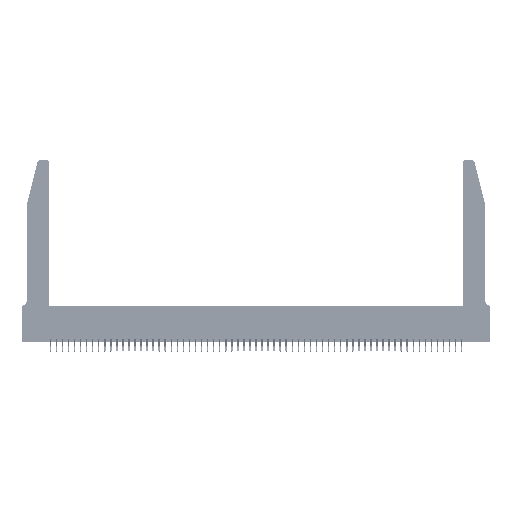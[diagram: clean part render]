
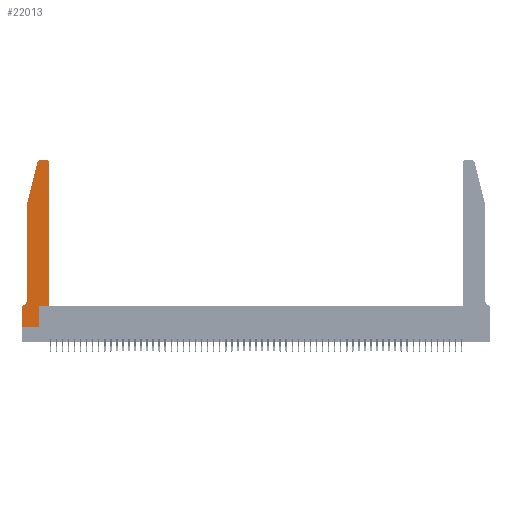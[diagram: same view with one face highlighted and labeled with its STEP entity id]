
A CAD part, top view. The second image highlights one B-rep face of the part: STEP entity #22013.
In plain terms, the highlighted planar face has unit normal (0, 0, 1).
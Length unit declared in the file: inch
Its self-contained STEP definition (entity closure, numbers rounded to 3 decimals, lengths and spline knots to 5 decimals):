
#356 = VERTEX_POINT ( 'NONE', #2509 ) ;
#990 = DIRECTION ( 'NONE',  ( 1., 0., 0. ) ) ;
#1100 = VECTOR ( 'NONE', #45764, 39.37008 ) ;
#1460 = FACE_OUTER_BOUND ( 'NONE', #21154, .T. ) ;
#1611 = EDGE_CURVE ( 'NONE', #2036, #16773, #53618, .T. ) ;
#2021 = CARTESIAN_POINT ( 'NONE',  ( 0.4205, 2.72, 0.37 ) ) ;
#2036 = VERTEX_POINT ( 'NONE', #11201 ) ;
#2509 = CARTESIAN_POINT ( 'NONE',  ( 0.4205, 2.75, 0.37 ) ) ;
#2712 = VERTEX_POINT ( 'NONE', #33238 ) ;
#3238 = AXIS2_PLACEMENT_3D ( 'NONE', #2021, #19494, #23577 ) ;
#3322 = EDGE_CURVE ( 'NONE', #19929, #51509, #54099, .T. ) ;
#5068 = DIRECTION ( 'NONE',  ( 1., 0., 0. ) ) ;
#5311 = VECTOR ( 'NONE', #25416, 39.37008 ) ;
#6392 = ORIENTED_EDGE ( 'NONE', *, *, #15690, .T. ) ;
#7091 = DIRECTION ( 'NONE',  ( 0., 0., -1. ) ) ;
#8102 = CARTESIAN_POINT ( 'NONE',  ( 0., 0., 0.37 ) ) ;
#8449 = VECTOR ( 'NONE', #48257, 39.37008 ) ;
#8916 = AXIS2_PLACEMENT_3D ( 'NONE', #30187, #37938, #5068 ) ;
#9371 = DIRECTION ( 'NONE',  ( 0., 0., 1. ) ) ;
#9622 = LINE ( 'NONE', #15098, #36476 ) ;
#9813 = CARTESIAN_POINT ( 'NONE',  ( 0.0755, 0.42, 0.37 ) ) ;
#11201 = CARTESIAN_POINT ( 'NONE',  ( 0.284, 2.75, 0.37 ) ) ;
#11797 = CIRCLE ( 'NONE', #3238, 0.03 ) ;
#12936 = ORIENTED_EDGE ( 'NONE', *, *, #1611, .T. ) ;
#13757 = VECTOR ( 'NONE', #17119, 39.37008 ) ;
#13805 = CARTESIAN_POINT ( 'NONE',  ( 0., 0., 0.37 ) ) ;
#14184 = ORIENTED_EDGE ( 'NONE', *, *, #43779, .T. ) ;
#14401 = EDGE_CURVE ( 'NONE', #19626, #46285, #19315, .T. ) ;
#14426 = CARTESIAN_POINT ( 'NONE',  ( 0.4505, 0.35, 0.37 ) ) ;
#14918 = ORIENTED_EDGE ( 'NONE', *, *, #39832, .T. ) ;
#15098 = CARTESIAN_POINT ( 'NONE',  ( 0.0755, 2., 0.37 ) ) ;
#15667 = EDGE_CURVE ( 'NONE', #20164, #30336, #42091, .T. ) ;
#15690 = EDGE_CURVE ( 'NONE', #51509, #20164, #54105, .T. ) ;
#16287 = CARTESIAN_POINT ( 'NONE',  ( 0.2865, 0., 0.37 ) ) ;
#16773 = VERTEX_POINT ( 'NONE', #22123 ) ;
#16777 = DIRECTION ( 'NONE',  ( -1., 0., 0. ) ) ;
#17119 = DIRECTION ( 'NONE',  ( -1., 0., 0. ) ) ;
#17463 = ORIENTED_EDGE ( 'NONE', *, *, #53093, .T. ) ;
#18027 = DIRECTION ( 'NONE',  ( 1., 0., 0. ) ) ;
#19315 = CIRCLE ( 'NONE', #42647, 0.07 ) ;
#19494 = DIRECTION ( 'NONE',  ( 0., 0., 1. ) ) ;
#19626 = VERTEX_POINT ( 'NONE', #9813 ) ;
#19929 = VERTEX_POINT ( 'NONE', #8102 ) ;
#20041 = CARTESIAN_POINT ( 'NONE',  ( 0.0055, 0.42, 0.37 ) ) ;
#20164 = VERTEX_POINT ( 'NONE', #22309 ) ;
#20710 = ORIENTED_EDGE ( 'NONE', *, *, #14401, .T. ) ;
#20864 = VERTEX_POINT ( 'NONE', #27313 ) ;
#21154 = EDGE_LOOP ( 'NONE', ( #17463, #12936, #31244, #14184, #20710, #14918, #38881, #27849, #6392, #27817, #22929, #31417 ) ) ;
#22013 = ADVANCED_FACE ( 'NONE', ( #1460 ), #30002, .T. ) ;
#22123 = CARTESIAN_POINT ( 'NONE',  ( 0.25487, 2.72718, 0.37 ) ) ;
#22309 = CARTESIAN_POINT ( 'NONE',  ( 0.2865, 0.35, 0.37 ) ) ;
#22929 = ORIENTED_EDGE ( 'NONE', *, *, #34795, .T. ) ;
#23577 = DIRECTION ( 'NONE',  ( 1., 0., 0. ) ) ;
#23970 = DIRECTION ( 'NONE',  ( -1., 0., 0. ) ) ;
#24467 = LINE ( 'NONE', #38311, #13757 ) ;
#24511 = LINE ( 'NONE', #13805, #8449 ) ;
#25411 = VECTOR ( 'NONE', #27321, 39.37008 ) ;
#25416 = DIRECTION ( 'NONE',  ( -0.239, -0.971, 0. ) ) ;
#26502 = CARTESIAN_POINT ( 'NONE',  ( 0.2865, 0.35, 0.37 ) ) ;
#27313 = CARTESIAN_POINT ( 'NONE',  ( 0.0755, 2., 0.37 ) ) ;
#27321 = DIRECTION ( 'NONE',  ( 0., 1., 0. ) ) ;
#27817 = ORIENTED_EDGE ( 'NONE', *, *, #15667, .T. ) ;
#27849 = ORIENTED_EDGE ( 'NONE', *, *, #3322, .T. ) ;
#30002 = PLANE ( 'NONE',  #8916 ) ;
#30187 = CARTESIAN_POINT ( 'NONE',  ( 0., 0.35, 0.37 ) ) ;
#30336 = VERTEX_POINT ( 'NONE', #43907 ) ;
#31244 = ORIENTED_EDGE ( 'NONE', *, *, #46100, .T. ) ;
#31417 = ORIENTED_EDGE ( 'NONE', *, *, #48821, .T. ) ;
#31618 = CARTESIAN_POINT ( 'NONE',  ( 0.4505, 2.72, 0.37 ) ) ;
#33238 = CARTESIAN_POINT ( 'NONE',  ( 0., 0.35, 0.37 ) ) ;
#34795 = EDGE_CURVE ( 'NONE', #30336, #46918, #49549, .T. ) ;
#35066 = CARTESIAN_POINT ( 'NONE',  ( 0.284, 2.72, 0.37 ) ) ;
#35327 = DIRECTION ( 'NONE',  ( 0., 1., 0. ) ) ;
#36059 = VECTOR ( 'NONE', #990, 39.37008 ) ;
#36476 = VECTOR ( 'NONE', #49364, 39.37008 ) ;
#37938 = DIRECTION ( 'NONE',  ( 0., 0., 1. ) ) ;
#37979 = EDGE_CURVE ( 'NONE', #2712, #19929, #24511, .T. ) ;
#38011 = CARTESIAN_POINT ( 'NONE',  ( 0.0755, 2., 0.37 ) ) ;
#38311 = CARTESIAN_POINT ( 'NONE',  ( 0.2605, 2.75, 0.37 ) ) ;
#38881 = ORIENTED_EDGE ( 'NONE', *, *, #37979, .T. ) ;
#39832 = EDGE_CURVE ( 'NONE', #46285, #2712, #53154, .T. ) ;
#42091 = LINE ( 'NONE', #52557, #36059 ) ;
#42222 = CARTESIAN_POINT ( 'NONE',  ( 0., 0., 0.37 ) ) ;
#42626 = CARTESIAN_POINT ( 'NONE',  ( 0.0755, 0.35, 0.37 ) ) ;
#42647 = AXIS2_PLACEMENT_3D ( 'NONE', #20041, #7091, #23970 ) ;
#43238 = CARTESIAN_POINT ( 'NONE',  ( 0.0055, 0.35, 0.37 ) ) ;
#43779 = EDGE_CURVE ( 'NONE', #20864, #19626, #9622, .T. ) ;
#43907 = CARTESIAN_POINT ( 'NONE',  ( 0.4505, 0.35, 0.37 ) ) ;
#45764 = DIRECTION ( 'NONE',  ( 1., 0., 0. ) ) ;
#46100 = EDGE_CURVE ( 'NONE', #16773, #20864, #48246, .T. ) ;
#46285 = VERTEX_POINT ( 'NONE', #43238 ) ;
#46918 = VERTEX_POINT ( 'NONE', #31618 ) ;
#47442 = VECTOR ( 'NONE', #35327, 39.37008 ) ;
#48246 = LINE ( 'NONE', #38011, #5311 ) ;
#48257 = DIRECTION ( 'NONE',  ( 0., -1., 0. ) ) ;
#48821 = EDGE_CURVE ( 'NONE', #46918, #356, #11797, .T. ) ;
#49106 = VECTOR ( 'NONE', #16777, 39.37008 ) ;
#49364 = DIRECTION ( 'NONE',  ( 0., -1., 0. ) ) ;
#49549 = LINE ( 'NONE', #14426, #25411 ) ;
#49748 = AXIS2_PLACEMENT_3D ( 'NONE', #35066, #9371, #18027 ) ;
#51509 = VERTEX_POINT ( 'NONE', #16287 ) ;
#52557 = CARTESIAN_POINT ( 'NONE',  ( 0.4505, 0.35, 0.37 ) ) ;
#53093 = EDGE_CURVE ( 'NONE', #356, #2036, #24467, .T. ) ;
#53154 = LINE ( 'NONE', #42626, #49106 ) ;
#53618 = CIRCLE ( 'NONE', #49748, 0.03 ) ;
#54099 = LINE ( 'NONE', #42222, #1100 ) ;
#54105 = LINE ( 'NONE', #26502, #47442 ) ;
